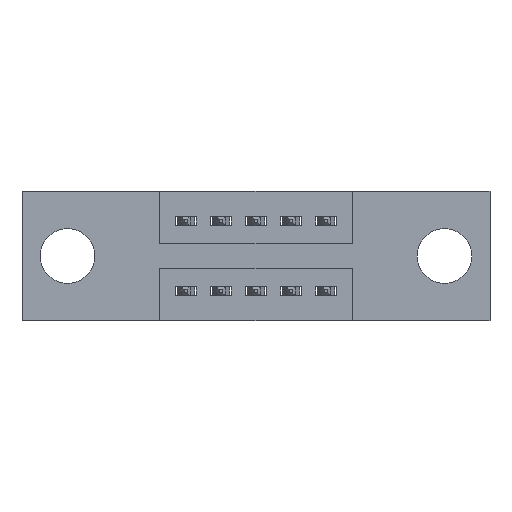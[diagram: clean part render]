
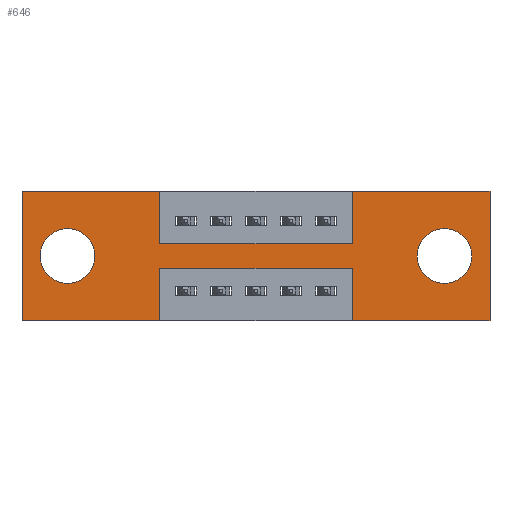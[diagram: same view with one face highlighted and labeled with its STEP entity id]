
A CAD part, front view. The second image highlights one B-rep face of the part: STEP entity #646.
In plain terms, the highlighted planar face has unit normal (0, -1, 0).
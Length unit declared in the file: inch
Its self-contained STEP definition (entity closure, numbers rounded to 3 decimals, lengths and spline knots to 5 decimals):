
#231 = EDGE_CURVE ( 'NONE', #6908, #2730, #3141, .T. ) ;
#316 = LINE ( 'NONE', #5241, #435 ) ;
#396 = CARTESIAN_POINT ( 'NONE',  ( 1.335, 0., 0. ) ) ;
#435 = VECTOR ( 'NONE', #8129, 39.37008 ) ;
#436 = CARTESIAN_POINT ( 'NONE',  ( 0., 0., 0. ) ) ;
#453 = VECTOR ( 'NONE', #2900, 39.37008 ) ;
#493 = FACE_BOUND ( 'NONE', #2738, .T. ) ;
#533 = DIRECTION ( 'NONE',  ( 0., 0., 1. ) ) ;
#646 = ADVANCED_FACE ( 'NONE', ( #493, #2666, #7830 ), #4936, .T. ) ;
#653 = CARTESIAN_POINT ( 'NONE',  ( 0.3925, 0., -0.22 ) ) ;
#688 = DIRECTION ( 'NONE',  ( 0., 0., -1. ) ) ;
#704 = EDGE_CURVE ( 'NONE', #6499, #4908, #8533, .T. ) ;
#759 = ORIENTED_EDGE ( 'NONE', *, *, #1981, .F. ) ;
#787 = VERTEX_POINT ( 'NONE', #3710 ) ;
#879 = EDGE_CURVE ( 'NONE', #5416, #2346, #1145, .T. ) ;
#1053 = CARTESIAN_POINT ( 'NONE',  ( 0.3925, 0., -0.15 ) ) ;
#1074 = VECTOR ( 'NONE', #3424, 39.37008 ) ;
#1145 = LINE ( 'NONE', #1053, #7179 ) ;
#1153 = ORIENTED_EDGE ( 'NONE', *, *, #7132, .F. ) ;
#1256 = CARTESIAN_POINT ( 'NONE',  ( 0., 0., 0. ) ) ;
#1432 = VERTEX_POINT ( 'NONE', #6869 ) ;
#1589 = AXIS2_PLACEMENT_3D ( 'NONE', #5884, #5181, #2289 ) ;
#1679 = ORIENTED_EDGE ( 'NONE', *, *, #3704, .F. ) ;
#1720 = DIRECTION ( 'NONE',  ( 1., 0., 0. ) ) ;
#1881 = ORIENTED_EDGE ( 'NONE', *, *, #6839, .T. ) ;
#1963 = DIRECTION ( 'NONE',  ( 0., -1., 0. ) ) ;
#1981 = EDGE_CURVE ( 'NONE', #2730, #5998, #5523, .T. ) ;
#2018 = LINE ( 'NONE', #6371, #6635 ) ;
#2117 = ORIENTED_EDGE ( 'NONE', *, *, #2599, .T. ) ;
#2289 = DIRECTION ( 'NONE',  ( 0., 0., 1. ) ) ;
#2346 = VERTEX_POINT ( 'NONE', #5594 ) ;
#2356 = ORIENTED_EDGE ( 'NONE', *, *, #2711, .F. ) ;
#2550 = VERTEX_POINT ( 'NONE', #6135 ) ;
#2566 = CIRCLE ( 'NONE', #6045, 0.078 ) ;
#2599 = EDGE_CURVE ( 'NONE', #4908, #6499, #3692, .T. ) ;
#2666 = FACE_BOUND ( 'NONE', #6591, .T. ) ;
#2711 = EDGE_CURVE ( 'NONE', #7146, #6908, #4189, .T. ) ;
#2730 = VERTEX_POINT ( 'NONE', #5655 ) ;
#2738 = EDGE_LOOP ( 'NONE', ( #1881, #7806 ) ) ;
#2900 = DIRECTION ( 'NONE',  ( -1., 0., 0. ) ) ;
#3098 = CARTESIAN_POINT ( 'NONE',  ( 1.335, 0., 0. ) ) ;
#3141 = LINE ( 'NONE', #396, #7089 ) ;
#3142 = EDGE_CURVE ( 'NONE', #2346, #7146, #6313, .T. ) ;
#3334 = CARTESIAN_POINT ( 'NONE',  ( 0.13, 0., -0.185 ) ) ;
#3424 = DIRECTION ( 'NONE',  ( 0., 0., -1. ) ) ;
#3468 = LINE ( 'NONE', #6404, #1074 ) ;
#3506 = CARTESIAN_POINT ( 'NONE',  ( 0., 0., 0. ) ) ;
#3578 = CARTESIAN_POINT ( 'NONE',  ( 1.205, 0., -0.185 ) ) ;
#3692 = CIRCLE ( 'NONE', #9125, 0.078 ) ;
#3697 = DIRECTION ( 'NONE',  ( 0., 1., 0. ) ) ;
#3704 = EDGE_CURVE ( 'NONE', #5930, #1432, #8527, .T. ) ;
#3710 = CARTESIAN_POINT ( 'NONE',  ( 0., 0., -0.37 ) ) ;
#3766 = VECTOR ( 'NONE', #4795, 39.37008 ) ;
#4038 = CARTESIAN_POINT ( 'NONE',  ( 0.3925, 0., -0.22 ) ) ;
#4061 = EDGE_CURVE ( 'NONE', #5964, #7477, #4916, .T. ) ;
#4105 = DIRECTION ( 'NONE',  ( 0., 1., 0. ) ) ;
#4141 = DIRECTION ( 'NONE',  ( 0., 0., -1. ) ) ;
#4189 = LINE ( 'NONE', #1256, #5504 ) ;
#4248 = ORIENTED_EDGE ( 'NONE', *, *, #8322, .F. ) ;
#4441 = VERTEX_POINT ( 'NONE', #8328 ) ;
#4529 = EDGE_CURVE ( 'NONE', #7477, #7076, #2018, .T. ) ;
#4692 = CIRCLE ( 'NONE', #7725, 0.078 ) ;
#4742 = AXIS2_PLACEMENT_3D ( 'NONE', #8580, #1963, #4141 ) ;
#4795 = DIRECTION ( 'NONE',  ( 0., 0., 1. ) ) ;
#4846 = EDGE_CURVE ( 'NONE', #787, #5930, #6169, .T. ) ;
#4876 = EDGE_CURVE ( 'NONE', #5998, #5964, #5548, .T. ) ;
#4891 = CARTESIAN_POINT ( 'NONE',  ( 0.9425, 0., 0. ) ) ;
#4908 = VERTEX_POINT ( 'NONE', #6885 ) ;
#4916 = LINE ( 'NONE', #653, #6937 ) ;
#4919 = ORIENTED_EDGE ( 'NONE', *, *, #3142, .F. ) ;
#4936 = PLANE ( 'NONE',  #4742 ) ;
#5147 = CARTESIAN_POINT ( 'NONE',  ( 0.9425, 0., -0.37 ) ) ;
#5151 = EDGE_LOOP ( 'NONE', ( #6767, #6426, #8410, #759, #8212, #2356, #4919, #6687, #1153, #1679, #7989, #4248 ) ) ;
#5181 = DIRECTION ( 'NONE',  ( 0., 1., 0. ) ) ;
#5189 = VECTOR ( 'NONE', #533, 39.37008 ) ;
#5241 = CARTESIAN_POINT ( 'NONE',  ( 0., 0., -0.37 ) ) ;
#5416 = VERTEX_POINT ( 'NONE', #5817 ) ;
#5472 = CARTESIAN_POINT ( 'NONE',  ( 0.9425, 0., 0. ) ) ;
#5504 = VECTOR ( 'NONE', #7078, 39.37008 ) ;
#5523 = LINE ( 'NONE', #9334, #453 ) ;
#5548 = LINE ( 'NONE', #7022, #5189 ) ;
#5561 = ORIENTED_EDGE ( 'NONE', *, *, #704, .T. ) ;
#5594 = CARTESIAN_POINT ( 'NONE',  ( 0.9425, 0., -0.15 ) ) ;
#5655 = CARTESIAN_POINT ( 'NONE',  ( 1.335, 0., -0.37 ) ) ;
#5817 = CARTESIAN_POINT ( 'NONE',  ( 0.3925, 0., -0.15 ) ) ;
#5884 = CARTESIAN_POINT ( 'NONE',  ( 0.13, 0., -0.185 ) ) ;
#5930 = VERTEX_POINT ( 'NONE', #8644 ) ;
#5964 = VERTEX_POINT ( 'NONE', #8788 ) ;
#5998 = VERTEX_POINT ( 'NONE', #5147 ) ;
#6020 = VECTOR ( 'NONE', #8622, 39.37008 ) ;
#6045 = AXIS2_PLACEMENT_3D ( 'NONE', #8055, #3697, #7445 ) ;
#6082 = DIRECTION ( 'NONE',  ( 0., 0., -1. ) ) ;
#6135 = CARTESIAN_POINT ( 'NONE',  ( 1.205, 0., -0.263 ) ) ;
#6169 = LINE ( 'NONE', #436, #3766 ) ;
#6313 = LINE ( 'NONE', #5472, #8979 ) ;
#6371 = CARTESIAN_POINT ( 'NONE',  ( 0.3925, 0., -0.37 ) ) ;
#6404 = CARTESIAN_POINT ( 'NONE',  ( 0.3925, 0., 0. ) ) ;
#6426 = ORIENTED_EDGE ( 'NONE', *, *, #4061, .F. ) ;
#6499 = VERTEX_POINT ( 'NONE', #6509 ) ;
#6509 = CARTESIAN_POINT ( 'NONE',  ( 0.13, 0., -0.263 ) ) ;
#6591 = EDGE_LOOP ( 'NONE', ( #2117, #5561 ) ) ;
#6635 = VECTOR ( 'NONE', #688, 39.37008 ) ;
#6687 = ORIENTED_EDGE ( 'NONE', *, *, #879, .F. ) ;
#6767 = ORIENTED_EDGE ( 'NONE', *, *, #4529, .F. ) ;
#6822 = DIRECTION ( 'NONE',  ( 0., 0., 1. ) ) ;
#6839 = EDGE_CURVE ( 'NONE', #4441, #2550, #4692, .T. ) ;
#6869 = CARTESIAN_POINT ( 'NONE',  ( 0.3925, 0., 0. ) ) ;
#6885 = CARTESIAN_POINT ( 'NONE',  ( 0.13, 0., -0.107 ) ) ;
#6908 = VERTEX_POINT ( 'NONE', #3098 ) ;
#6937 = VECTOR ( 'NONE', #8471, 39.37008 ) ;
#7022 = CARTESIAN_POINT ( 'NONE',  ( 0.9425, 0., -0.37 ) ) ;
#7076 = VERTEX_POINT ( 'NONE', #7829 ) ;
#7078 = DIRECTION ( 'NONE',  ( 1., 0., 0. ) ) ;
#7089 = VECTOR ( 'NONE', #6082, 39.37008 ) ;
#7132 = EDGE_CURVE ( 'NONE', #1432, #5416, #3468, .T. ) ;
#7146 = VERTEX_POINT ( 'NONE', #4891 ) ;
#7179 = VECTOR ( 'NONE', #1720, 39.37008 ) ;
#7445 = DIRECTION ( 'NONE',  ( 0., 0., -1. ) ) ;
#7477 = VERTEX_POINT ( 'NONE', #4038 ) ;
#7655 = DIRECTION ( 'NONE',  ( 0., 0., 1. ) ) ;
#7725 = AXIS2_PLACEMENT_3D ( 'NONE', #3578, #9354, #8874 ) ;
#7759 = EDGE_CURVE ( 'NONE', #2550, #4441, #2566, .T. ) ;
#7806 = ORIENTED_EDGE ( 'NONE', *, *, #7759, .T. ) ;
#7829 = CARTESIAN_POINT ( 'NONE',  ( 0.3925, 0., -0.37 ) ) ;
#7830 = FACE_OUTER_BOUND ( 'NONE', #5151, .T. ) ;
#7989 = ORIENTED_EDGE ( 'NONE', *, *, #4846, .F. ) ;
#8055 = CARTESIAN_POINT ( 'NONE',  ( 1.205, 0., -0.185 ) ) ;
#8129 = DIRECTION ( 'NONE',  ( -1., 0., 0. ) ) ;
#8212 = ORIENTED_EDGE ( 'NONE', *, *, #231, .F. ) ;
#8322 = EDGE_CURVE ( 'NONE', #7076, #787, #316, .T. ) ;
#8328 = CARTESIAN_POINT ( 'NONE',  ( 1.205, 0., -0.107 ) ) ;
#8410 = ORIENTED_EDGE ( 'NONE', *, *, #4876, .F. ) ;
#8471 = DIRECTION ( 'NONE',  ( -1., 0., 0. ) ) ;
#8527 = LINE ( 'NONE', #3506, #6020 ) ;
#8533 = CIRCLE ( 'NONE', #1589, 0.078 ) ;
#8580 = CARTESIAN_POINT ( 'NONE',  ( 0., 0., -0.37 ) ) ;
#8622 = DIRECTION ( 'NONE',  ( 1., 0., 0. ) ) ;
#8644 = CARTESIAN_POINT ( 'NONE',  ( 0., 0., 0. ) ) ;
#8788 = CARTESIAN_POINT ( 'NONE',  ( 0.9425, 0., -0.22 ) ) ;
#8874 = DIRECTION ( 'NONE',  ( 0., 0., -1. ) ) ;
#8979 = VECTOR ( 'NONE', #7655, 39.37008 ) ;
#9125 = AXIS2_PLACEMENT_3D ( 'NONE', #3334, #4105, #6822 ) ;
#9334 = CARTESIAN_POINT ( 'NONE',  ( 0., 0., -0.37 ) ) ;
#9354 = DIRECTION ( 'NONE',  ( 0., 1., 0. ) ) ;
